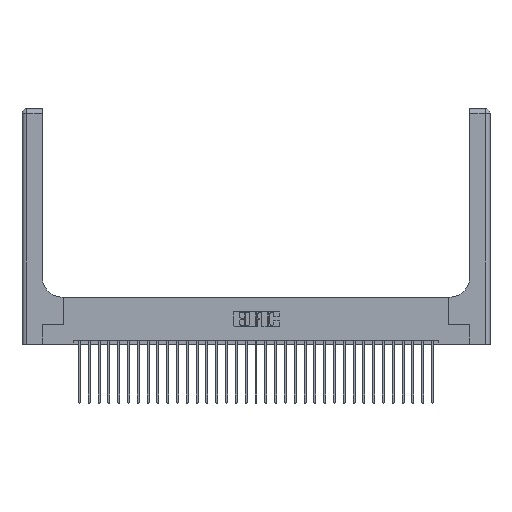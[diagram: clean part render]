
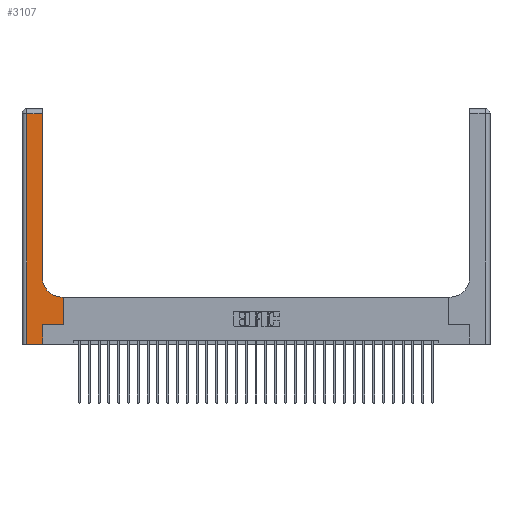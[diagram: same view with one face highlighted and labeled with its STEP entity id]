
A CAD part, top view. The second image highlights one B-rep face of the part: STEP entity #3107.
In plain terms, the highlighted planar face has unit normal (0, 0, 1).
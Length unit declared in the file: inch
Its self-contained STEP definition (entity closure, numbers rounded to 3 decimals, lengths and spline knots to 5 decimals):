
#62 = VERTEX_POINT ( 'NONE', #29313 ) ;
#2315 = EDGE_LOOP ( 'NONE', ( #8795, #24053, #7729, #23876, #21520, #16903, #27744, #14557, #22148 ) ) ;
#2362 = LINE ( 'NONE', #9318, #9390 ) ;
#2637 = DIRECTION ( 'NONE',  ( 1., 0., 0. ) ) ;
#2966 = CARTESIAN_POINT ( 'NONE',  ( 0.26, 0.85, 0.37 ) ) ;
#3107 = ADVANCED_FACE ( 'NONE', ( #29288 ), #24841, .F. ) ;
#3696 = CARTESIAN_POINT ( 'NONE',  ( 0., 3., 0.37 ) ) ;
#3782 = VECTOR ( 'NONE', #24136, 39.37008 ) ;
#4008 = CARTESIAN_POINT ( 'NONE',  ( 0., 0., 0.37 ) ) ;
#4669 = EDGE_CURVE ( 'NONE', #25158, #28091, #6776, .T. ) ;
#6548 = CARTESIAN_POINT ( 'NONE',  ( 0.06, 2.94, 0.37 ) ) ;
#6776 = LINE ( 'NONE', #18217, #20443 ) ;
#7021 = DIRECTION ( 'NONE',  ( -1., 0., 0. ) ) ;
#7729 = ORIENTED_EDGE ( 'NONE', *, *, #23028, .T. ) ;
#8003 = EDGE_CURVE ( 'NONE', #28091, #29786, #30177, .T. ) ;
#8520 = VERTEX_POINT ( 'NONE', #26417 ) ;
#8710 = DIRECTION ( 'NONE',  ( 1., 0., 0. ) ) ;
#8795 = ORIENTED_EDGE ( 'NONE', *, *, #4669, .T. ) ;
#9069 = CARTESIAN_POINT ( 'NONE',  ( 0.265, 0., 0.37 ) ) ;
#9318 = CARTESIAN_POINT ( 'NONE',  ( 0.06, 3., 0.37 ) ) ;
#9390 = VECTOR ( 'NONE', #14240, 39.37008 ) ;
#9596 = LINE ( 'NONE', #19624, #11084 ) ;
#9976 = CARTESIAN_POINT ( 'NONE',  ( 0.528, 0.25, 0.37 ) ) ;
#10391 = EDGE_CURVE ( 'NONE', #20919, #17750, #13868, .T. ) ;
#10559 = DIRECTION ( 'NONE',  ( 0., 0., -1. ) ) ;
#11084 = VECTOR ( 'NONE', #2637, 39.37008 ) ;
#12237 = EDGE_CURVE ( 'NONE', #23190, #20919, #9596, .T. ) ;
#12406 = EDGE_CURVE ( 'NONE', #62, #29679, #15733, .T. ) ;
#12673 = CARTESIAN_POINT ( 'NONE',  ( 0.265, 0.25, 0.37 ) ) ;
#13098 = DIRECTION ( 'NONE',  ( -1., 0., 0. ) ) ;
#13373 = VECTOR ( 'NONE', #25297, 39.37008 ) ;
#13494 = CARTESIAN_POINT ( 'NONE',  ( 0.265, 0., 0.37 ) ) ;
#13561 = DIRECTION ( 'NONE',  ( 0., 1., 0. ) ) ;
#13687 = DIRECTION ( 'NONE',  ( 0., 1., 0. ) ) ;
#13868 = LINE ( 'NONE', #23301, #13373 ) ;
#14148 = CARTESIAN_POINT ( 'NONE',  ( 0.26, 2.94, 0.37 ) ) ;
#14240 = DIRECTION ( 'NONE',  ( 0., -1., 0. ) ) ;
#14557 = ORIENTED_EDGE ( 'NONE', *, *, #16990, .T. ) ;
#15733 = LINE ( 'NONE', #4008, #20041 ) ;
#16003 = LINE ( 'NONE', #9069, #17161 ) ;
#16856 = CIRCLE ( 'NONE', #24258, 0.25 ) ;
#16903 = ORIENTED_EDGE ( 'NONE', *, *, #12237, .T. ) ;
#16990 = EDGE_CURVE ( 'NONE', #17750, #8520, #27041, .T. ) ;
#17161 = VECTOR ( 'NONE', #13687, 39.37008 ) ;
#17750 = VERTEX_POINT ( 'NONE', #21322 ) ;
#17828 = CARTESIAN_POINT ( 'NONE',  ( 0.51, 0.85, 0.37 ) ) ;
#17851 = AXIS2_PLACEMENT_3D ( 'NONE', #3696, #26986, #13098 ) ;
#18217 = CARTESIAN_POINT ( 'NONE',  ( 0.26, 3., 0.37 ) ) ;
#19624 = CARTESIAN_POINT ( 'NONE',  ( 0.265, 0.25, 0.37 ) ) ;
#20041 = VECTOR ( 'NONE', #22377, 39.37008 ) ;
#20443 = VECTOR ( 'NONE', #13561, 39.37008 ) ;
#20808 = EDGE_CURVE ( 'NONE', #29679, #23190, #16003, .T. ) ;
#20919 = VERTEX_POINT ( 'NONE', #9976 ) ;
#21322 = CARTESIAN_POINT ( 'NONE',  ( 0.528, 0.6, 0.37 ) ) ;
#21520 = ORIENTED_EDGE ( 'NONE', *, *, #20808, .T. ) ;
#21833 = CARTESIAN_POINT ( 'NONE',  ( 0.26, 0.6, 0.37 ) ) ;
#22148 = ORIENTED_EDGE ( 'NONE', *, *, #27399, .T. ) ;
#22377 = DIRECTION ( 'NONE',  ( 1., 0., 0. ) ) ;
#23028 = EDGE_CURVE ( 'NONE', #29786, #62, #2362, .T. ) ;
#23190 = VERTEX_POINT ( 'NONE', #12673 ) ;
#23301 = CARTESIAN_POINT ( 'NONE',  ( 0.528, 0.25, 0.37 ) ) ;
#23876 = ORIENTED_EDGE ( 'NONE', *, *, #12406, .T. ) ;
#24053 = ORIENTED_EDGE ( 'NONE', *, *, #8003, .T. ) ;
#24136 = DIRECTION ( 'NONE',  ( -1., 0., 0. ) ) ;
#24258 = AXIS2_PLACEMENT_3D ( 'NONE', #17828, #10559, #8710 ) ;
#24841 = PLANE ( 'NONE',  #17851 ) ;
#25158 = VERTEX_POINT ( 'NONE', #2966 ) ;
#25297 = DIRECTION ( 'NONE',  ( 0., 1., 0. ) ) ;
#26417 = CARTESIAN_POINT ( 'NONE',  ( 0.51, 0.6, 0.37 ) ) ;
#26986 = DIRECTION ( 'NONE',  ( 0., 0., -1. ) ) ;
#27041 = LINE ( 'NONE', #21833, #3782 ) ;
#27399 = EDGE_CURVE ( 'NONE', #8520, #25158, #16856, .T. ) ;
#27744 = ORIENTED_EDGE ( 'NONE', *, *, #10391, .T. ) ;
#28091 = VERTEX_POINT ( 'NONE', #14148 ) ;
#28457 = CARTESIAN_POINT ( 'NONE',  ( 0., 2.94, 0.37 ) ) ;
#29288 = FACE_OUTER_BOUND ( 'NONE', #2315, .T. ) ;
#29313 = CARTESIAN_POINT ( 'NONE',  ( 0.06, 0., 0.37 ) ) ;
#29582 = VECTOR ( 'NONE', #7021, 39.37008 ) ;
#29679 = VERTEX_POINT ( 'NONE', #13494 ) ;
#29786 = VERTEX_POINT ( 'NONE', #6548 ) ;
#30177 = LINE ( 'NONE', #28457, #29582 ) ;
